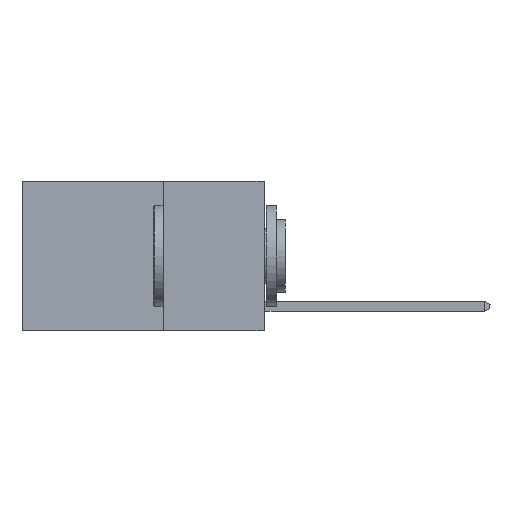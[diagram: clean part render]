
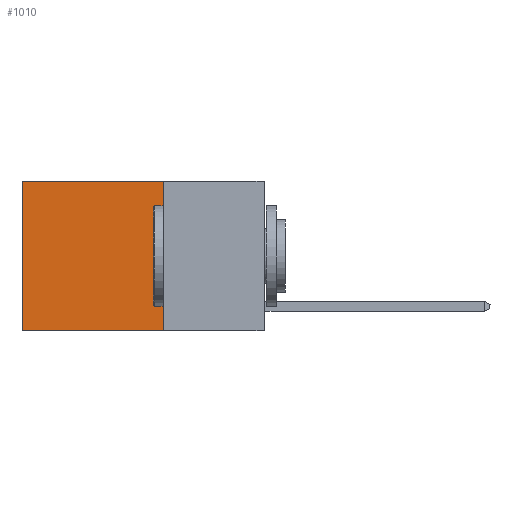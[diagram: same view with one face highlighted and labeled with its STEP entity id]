
A CAD part, left-side view. The second image highlights one B-rep face of the part: STEP entity #1010.
In plain terms, the highlighted planar face has unit normal (-1, 0, 0).
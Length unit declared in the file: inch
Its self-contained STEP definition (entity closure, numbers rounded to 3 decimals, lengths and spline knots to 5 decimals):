
#1010 = ADVANCED_FACE ( 'NONE', ( #2412 ), #1039, .F. ) ;
#1016 = VERTEX_POINT ( 'NONE', #7226 ) ;
#1039 = PLANE ( 'NONE',  #10016 ) ;
#1067 = ORIENTED_EDGE ( 'NONE', *, *, #8487, .F. ) ;
#1340 = VECTOR ( 'NONE', #10227, 39.37008 ) ;
#1509 = CARTESIAN_POINT ( 'NONE',  ( 0.2625, 0.6, 0. ) ) ;
#1518 = ORIENTED_EDGE ( 'NONE', *, *, #9196, .T. ) ;
#2223 = DIRECTION ( 'NONE',  ( 1., 0., 0. ) ) ;
#2412 = FACE_OUTER_BOUND ( 'NONE', #11125, .T. ) ;
#2952 = ORIENTED_EDGE ( 'NONE', *, *, #3661, .T. ) ;
#3035 = VECTOR ( 'NONE', #7228, 39.37008 ) ;
#3261 = EDGE_CURVE ( 'NONE', #11435, #7543, #4113, .T. ) ;
#3424 = CARTESIAN_POINT ( 'NONE',  ( 0.2625, 0.25, -0.37 ) ) ;
#3661 = EDGE_CURVE ( 'NONE', #1016, #9019, #9718, .T. ) ;
#3727 = DIRECTION ( 'NONE',  ( 0., 0., -1. ) ) ;
#3807 = VECTOR ( 'NONE', #5611, 39.37008 ) ;
#4113 = LINE ( 'NONE', #6784, #1340 ) ;
#4657 = CARTESIAN_POINT ( 'NONE',  ( 0.2625, 0.25, 0. ) ) ;
#5178 = VECTOR ( 'NONE', #3727, 39.37008 ) ;
#5189 = DIRECTION ( 'NONE',  ( 0., 0., -1. ) ) ;
#5611 = DIRECTION ( 'NONE',  ( 0., 1., 0. ) ) ;
#6784 = CARTESIAN_POINT ( 'NONE',  ( 0.2625, 0.25, 0. ) ) ;
#7226 = CARTESIAN_POINT ( 'NONE',  ( 0.2625, 0.6, 0. ) ) ;
#7228 = DIRECTION ( 'NONE',  ( 0., 1., 0. ) ) ;
#7543 = VERTEX_POINT ( 'NONE', #3424 ) ;
#8487 = EDGE_CURVE ( 'NONE', #7543, #9019, #11839, .T. ) ;
#9019 = VERTEX_POINT ( 'NONE', #11163 ) ;
#9196 = EDGE_CURVE ( 'NONE', #11435, #1016, #12452, .T. ) ;
#9224 = CARTESIAN_POINT ( 'NONE',  ( 0.2625, 0.25, -0.37 ) ) ;
#9638 = CARTESIAN_POINT ( 'NONE',  ( 0.2625, 0.25, 0. ) ) ;
#9718 = LINE ( 'NONE', #1509, #5178 ) ;
#10016 = AXIS2_PLACEMENT_3D ( 'NONE', #10098, #2223, #5189 ) ;
#10098 = CARTESIAN_POINT ( 'NONE',  ( 0.2625, 0.25, 0. ) ) ;
#10227 = DIRECTION ( 'NONE',  ( 0., 0., -1. ) ) ;
#11125 = EDGE_LOOP ( 'NONE', ( #2952, #1067, #11843, #1518 ) ) ;
#11163 = CARTESIAN_POINT ( 'NONE',  ( 0.2625, 0.6, -0.37 ) ) ;
#11435 = VERTEX_POINT ( 'NONE', #9638 ) ;
#11839 = LINE ( 'NONE', #9224, #3035 ) ;
#11843 = ORIENTED_EDGE ( 'NONE', *, *, #3261, .F. ) ;
#12452 = LINE ( 'NONE', #4657, #3807 ) ;
